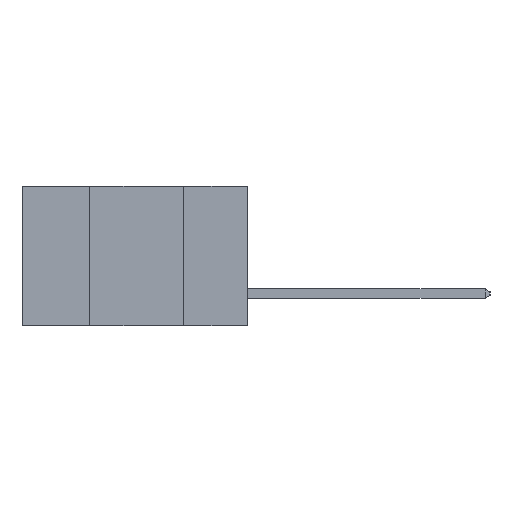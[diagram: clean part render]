
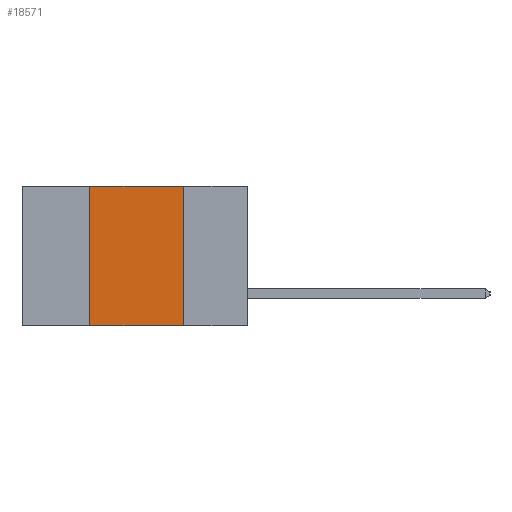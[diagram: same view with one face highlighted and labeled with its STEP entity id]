
A CAD part, left-side view. The second image highlights one B-rep face of the part: STEP entity #18571.
In plain terms, the highlighted planar face has unit normal (-1, 0, 0).
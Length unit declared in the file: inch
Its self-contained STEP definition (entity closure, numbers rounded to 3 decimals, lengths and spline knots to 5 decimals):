
#219 = VECTOR ( 'NONE', #10937, 39.37008 ) ;
#383 = ORIENTED_EDGE ( 'NONE', *, *, #6937, .F. ) ;
#2074 = CARTESIAN_POINT ( 'NONE',  ( 0., 0.6, 0. ) ) ;
#2084 = ORIENTED_EDGE ( 'NONE', *, *, #15716, .F. ) ;
#2400 = LINE ( 'NONE', #3459, #23216 ) ;
#3459 = CARTESIAN_POINT ( 'NONE',  ( 0., 0.17, 0. ) ) ;
#3880 = EDGE_CURVE ( 'NONE', #26674, #14304, #13462, .T. ) ;
#3993 = CARTESIAN_POINT ( 'NONE',  ( 0., 0.17, -0.37 ) ) ;
#5053 = ORIENTED_EDGE ( 'NONE', *, *, #21973, .T. ) ;
#5111 = LINE ( 'NONE', #20404, #11300 ) ;
#5792 = FACE_OUTER_BOUND ( 'NONE', #5998, .T. ) ;
#5998 = EDGE_LOOP ( 'NONE', ( #2084, #10904, #383, #5053 ) ) ;
#6937 = EDGE_CURVE ( 'NONE', #26104, #26674, #5111, .T. ) ;
#8358 = DIRECTION ( 'NONE',  ( 0., -1., 0. ) ) ;
#8431 = PLANE ( 'NONE',  #19558 ) ;
#10504 = DIRECTION ( 'NONE',  ( 0., 0., -1. ) ) ;
#10904 = ORIENTED_EDGE ( 'NONE', *, *, #3880, .F. ) ;
#10937 = DIRECTION ( 'NONE',  ( 0., -1., 0. ) ) ;
#11300 = VECTOR ( 'NONE', #12112, 39.37008 ) ;
#12112 = DIRECTION ( 'NONE',  ( 0., 0., 1. ) ) ;
#13462 = LINE ( 'NONE', #2074, #18360 ) ;
#14304 = VERTEX_POINT ( 'NONE', #17851 ) ;
#14639 = CARTESIAN_POINT ( 'NONE',  ( 0., 0.6, 0. ) ) ;
#15464 = CARTESIAN_POINT ( 'NONE',  ( 0., 0.42, 0. ) ) ;
#15716 = EDGE_CURVE ( 'NONE', #14304, #19833, #2400, .T. ) ;
#17851 = CARTESIAN_POINT ( 'NONE',  ( 0., 0.17, 0. ) ) ;
#18262 = LINE ( 'NONE', #25462, #219 ) ;
#18360 = VECTOR ( 'NONE', #8358, 39.37008 ) ;
#18571 = ADVANCED_FACE ( 'NONE', ( #5792 ), #8431, .F. ) ;
#19558 = AXIS2_PLACEMENT_3D ( 'NONE', #14639, #22960, #10504 ) ;
#19833 = VERTEX_POINT ( 'NONE', #3993 ) ;
#20404 = CARTESIAN_POINT ( 'NONE',  ( 0., 0.42, 0. ) ) ;
#21973 = EDGE_CURVE ( 'NONE', #26104, #19833, #18262, .T. ) ;
#22208 = DIRECTION ( 'NONE',  ( 0., 0., -1. ) ) ;
#22960 = DIRECTION ( 'NONE',  ( 1., 0., 0. ) ) ;
#23216 = VECTOR ( 'NONE', #22208, 39.37008 ) ;
#25462 = CARTESIAN_POINT ( 'NONE',  ( 0., 0.6, -0.37 ) ) ;
#25800 = CARTESIAN_POINT ( 'NONE',  ( 0., 0.42, -0.37 ) ) ;
#26104 = VERTEX_POINT ( 'NONE', #25800 ) ;
#26674 = VERTEX_POINT ( 'NONE', #15464 ) ;
